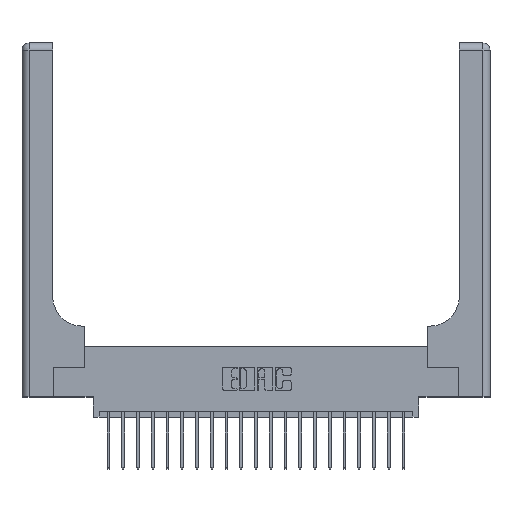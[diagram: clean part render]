
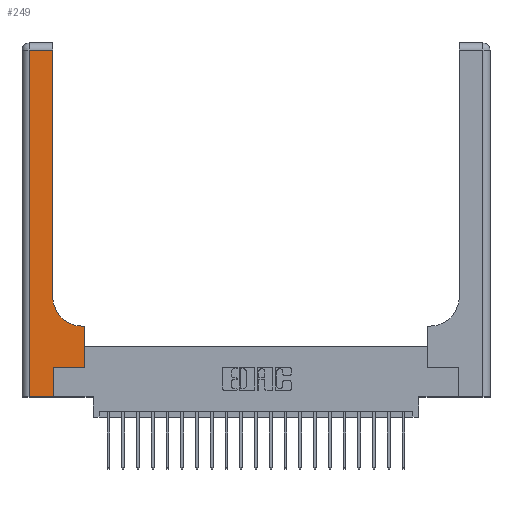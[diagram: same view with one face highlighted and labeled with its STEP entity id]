
A CAD part, top view. The second image highlights one B-rep face of the part: STEP entity #249.
In plain terms, the highlighted planar face has unit normal (0, 0, 1).
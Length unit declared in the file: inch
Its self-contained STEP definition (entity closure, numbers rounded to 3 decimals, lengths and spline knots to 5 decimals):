
#103 = FACE_OUTER_BOUND ( 'NONE', #14397, .T. ) ;
#226 = DIRECTION ( 'NONE',  ( 1., 0., 0. ) ) ;
#249 = ADVANCED_FACE ( 'NONE', ( #103 ), #15342, .F. ) ;
#326 = LINE ( 'NONE', #19620, #17789 ) ;
#471 = EDGE_CURVE ( 'NONE', #10974, #19172, #10391, .T. ) ;
#983 = ORIENTED_EDGE ( 'NONE', *, *, #6419, .T. ) ;
#1252 = CARTESIAN_POINT ( 'NONE',  ( 0.265, 0., 0.37 ) ) ;
#1884 = CARTESIAN_POINT ( 'NONE',  ( 0.528, 0.25, 0.37 ) ) ;
#1896 = ORIENTED_EDGE ( 'NONE', *, *, #7771, .T. ) ;
#2186 = CARTESIAN_POINT ( 'NONE',  ( 0.265, 0.25, 0.37 ) ) ;
#2677 = DIRECTION ( 'NONE',  ( 0., 1., 0. ) ) ;
#2751 = DIRECTION ( 'NONE',  ( 0., 1., 0. ) ) ;
#3164 = CARTESIAN_POINT ( 'NONE',  ( 0.528, 0.6, 0.37 ) ) ;
#3180 = AXIS2_PLACEMENT_3D ( 'NONE', #14887, #14199, #14150 ) ;
#3191 = CARTESIAN_POINT ( 'NONE',  ( 0.528, 0.25, 0.37 ) ) ;
#3253 = CIRCLE ( 'NONE', #5486, 0.25 ) ;
#3259 = ORIENTED_EDGE ( 'NONE', *, *, #15297, .T. ) ;
#3288 = CARTESIAN_POINT ( 'NONE',  ( 0.06, 2.94, 0.37 ) ) ;
#3442 = ORIENTED_EDGE ( 'NONE', *, *, #6962, .T. ) ;
#3500 = VERTEX_POINT ( 'NONE', #15271 ) ;
#3576 = CARTESIAN_POINT ( 'NONE',  ( 0.51, 0.6, 0.37 ) ) ;
#4003 = ORIENTED_EDGE ( 'NONE', *, *, #5610, .T. ) ;
#4579 = LINE ( 'NONE', #1252, #8502 ) ;
#4799 = VECTOR ( 'NONE', #20781, 39.37008 ) ;
#5052 = ORIENTED_EDGE ( 'NONE', *, *, #6178, .T. ) ;
#5071 = LINE ( 'NONE', #6182, #13991 ) ;
#5486 = AXIS2_PLACEMENT_3D ( 'NONE', #20501, #10319, #226 ) ;
#5610 = EDGE_CURVE ( 'NONE', #12275, #12406, #326, .T. ) ;
#6178 = EDGE_CURVE ( 'NONE', #19172, #13273, #5071, .T. ) ;
#6182 = CARTESIAN_POINT ( 'NONE',  ( 0.26, 0.6, 0.37 ) ) ;
#6272 = VERTEX_POINT ( 'NONE', #14860 ) ;
#6419 = EDGE_CURVE ( 'NONE', #10434, #6272, #18282, .T. ) ;
#6962 = EDGE_CURVE ( 'NONE', #12406, #10434, #21666, .T. ) ;
#7771 = EDGE_CURVE ( 'NONE', #3500, #10974, #19292, .T. ) ;
#8086 = ORIENTED_EDGE ( 'NONE', *, *, #21538, .T. ) ;
#8502 = VECTOR ( 'NONE', #9613, 39.37008 ) ;
#8982 = CARTESIAN_POINT ( 'NONE',  ( 0.26, 2.94, 0.37 ) ) ;
#9495 = DIRECTION ( 'NONE',  ( 1., 0., 0. ) ) ;
#9613 = DIRECTION ( 'NONE',  ( 0., 1., 0. ) ) ;
#9939 = LINE ( 'NONE', #21367, #14433 ) ;
#10319 = DIRECTION ( 'NONE',  ( 0., 0., -1. ) ) ;
#10391 = LINE ( 'NONE', #1884, #20498 ) ;
#10434 = VERTEX_POINT ( 'NONE', #3288 ) ;
#10974 = VERTEX_POINT ( 'NONE', #3191 ) ;
#12016 = CARTESIAN_POINT ( 'NONE',  ( 0., 2.94, 0.37 ) ) ;
#12275 = VERTEX_POINT ( 'NONE', #15329 ) ;
#12406 = VERTEX_POINT ( 'NONE', #8982 ) ;
#13273 = VERTEX_POINT ( 'NONE', #3576 ) ;
#13991 = VECTOR ( 'NONE', #16267, 39.37008 ) ;
#14150 = DIRECTION ( 'NONE',  ( -1., 0., 0. ) ) ;
#14199 = DIRECTION ( 'NONE',  ( 0., 0., -1. ) ) ;
#14397 = EDGE_LOOP ( 'NONE', ( #4003, #3442, #983, #20283, #8086, #1896, #15757, #5052, #3259 ) ) ;
#14433 = VECTOR ( 'NONE', #9495, 39.37008 ) ;
#14860 = CARTESIAN_POINT ( 'NONE',  ( 0.06, 0., 0.37 ) ) ;
#14887 = CARTESIAN_POINT ( 'NONE',  ( 0., 3., 0.37 ) ) ;
#15271 = CARTESIAN_POINT ( 'NONE',  ( 0.265, 0.25, 0.37 ) ) ;
#15297 = EDGE_CURVE ( 'NONE', #13273, #12275, #3253, .T. ) ;
#15329 = CARTESIAN_POINT ( 'NONE',  ( 0.26, 0.85, 0.37 ) ) ;
#15342 = PLANE ( 'NONE',  #3180 ) ;
#15757 = ORIENTED_EDGE ( 'NONE', *, *, #471, .T. ) ;
#16267 = DIRECTION ( 'NONE',  ( -1., 0., 0. ) ) ;
#17045 = VERTEX_POINT ( 'NONE', #18145 ) ;
#17153 = VECTOR ( 'NONE', #18921, 39.37008 ) ;
#17789 = VECTOR ( 'NONE', #2751, 39.37008 ) ;
#18145 = CARTESIAN_POINT ( 'NONE',  ( 0.265, 0., 0.37 ) ) ;
#18282 = LINE ( 'NONE', #19100, #4799 ) ;
#18333 = EDGE_CURVE ( 'NONE', #6272, #17045, #9939, .T. ) ;
#18921 = DIRECTION ( 'NONE',  ( -1., 0., 0. ) ) ;
#19100 = CARTESIAN_POINT ( 'NONE',  ( 0.06, 3., 0.37 ) ) ;
#19121 = DIRECTION ( 'NONE',  ( 1., 0., 0. ) ) ;
#19172 = VERTEX_POINT ( 'NONE', #3164 ) ;
#19292 = LINE ( 'NONE', #2186, #19835 ) ;
#19620 = CARTESIAN_POINT ( 'NONE',  ( 0.26, 3., 0.37 ) ) ;
#19835 = VECTOR ( 'NONE', #19121, 39.37008 ) ;
#20283 = ORIENTED_EDGE ( 'NONE', *, *, #18333, .T. ) ;
#20498 = VECTOR ( 'NONE', #2677, 39.37008 ) ;
#20501 = CARTESIAN_POINT ( 'NONE',  ( 0.51, 0.85, 0.37 ) ) ;
#20781 = DIRECTION ( 'NONE',  ( 0., -1., 0. ) ) ;
#21367 = CARTESIAN_POINT ( 'NONE',  ( 0., 0., 0.37 ) ) ;
#21538 = EDGE_CURVE ( 'NONE', #17045, #3500, #4579, .T. ) ;
#21666 = LINE ( 'NONE', #12016, #17153 ) ;
